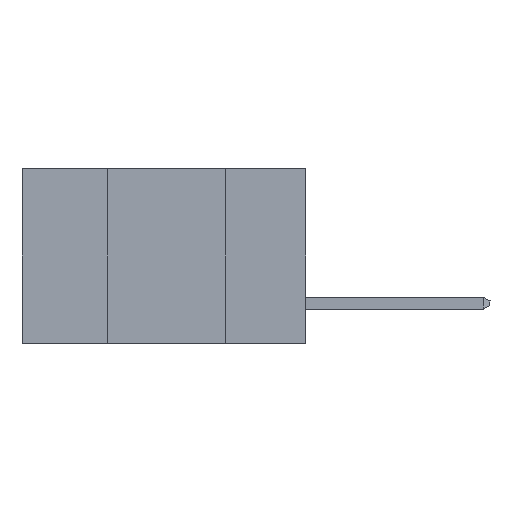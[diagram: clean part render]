
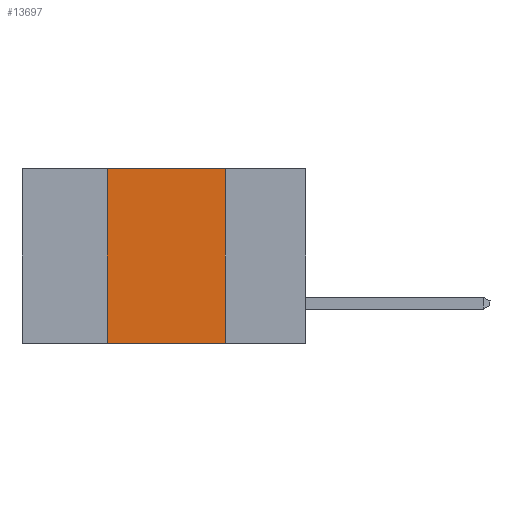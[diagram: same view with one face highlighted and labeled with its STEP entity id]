
A CAD part, left-side view. The second image highlights one B-rep face of the part: STEP entity #13697.
In plain terms, the highlighted planar face has unit normal (-1, 0, 0).
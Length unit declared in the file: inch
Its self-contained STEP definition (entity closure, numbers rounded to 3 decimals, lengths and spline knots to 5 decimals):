
#27 = VECTOR ( 'NONE', #10777, 39.37008 ) ;
#52 = DIRECTION ( 'NONE',  ( 0., -1., 0. ) ) ;
#496 = DIRECTION ( 'NONE',  ( 1., 0., 0. ) ) ;
#500 = DIRECTION ( 'NONE',  ( 0., 0., 1. ) ) ;
#2485 = EDGE_CURVE ( 'NONE', #3078, #5836, #11217, .T. ) ;
#2499 = ORIENTED_EDGE ( 'NONE', *, *, #14195, .F. ) ;
#2854 = VECTOR ( 'NONE', #4933, 39.37008 ) ;
#3003 = AXIS2_PLACEMENT_3D ( 'NONE', #12681, #496, #5812 ) ;
#3078 = VERTEX_POINT ( 'NONE', #17402 ) ;
#3918 = FACE_OUTER_BOUND ( 'NONE', #5797, .T. ) ;
#4214 = CARTESIAN_POINT ( 'NONE',  ( 0., 0.17, -0.37 ) ) ;
#4348 = LINE ( 'NONE', #12487, #27 ) ;
#4933 = DIRECTION ( 'NONE',  ( 0., 0., -1. ) ) ;
#5797 = EDGE_LOOP ( 'NONE', ( #2499, #14328, #10092, #8984 ) ) ;
#5812 = DIRECTION ( 'NONE',  ( 0., 0., -1. ) ) ;
#5836 = VERTEX_POINT ( 'NONE', #7734 ) ;
#6937 = CARTESIAN_POINT ( 'NONE',  ( 0., 0.17, 0. ) ) ;
#7551 = VECTOR ( 'NONE', #500, 39.37008 ) ;
#7584 = CARTESIAN_POINT ( 'NONE',  ( 0., 0.17, 0. ) ) ;
#7734 = CARTESIAN_POINT ( 'NONE',  ( 0., 0.42, 0. ) ) ;
#8492 = VERTEX_POINT ( 'NONE', #6937 ) ;
#8624 = EDGE_CURVE ( 'NONE', #3078, #15073, #16427, .T. ) ;
#8984 = ORIENTED_EDGE ( 'NONE', *, *, #8624, .T. ) ;
#10092 = ORIENTED_EDGE ( 'NONE', *, *, #2485, .F. ) ;
#10193 = LINE ( 'NONE', #7584, #2854 ) ;
#10777 = DIRECTION ( 'NONE',  ( 0., -1., 0. ) ) ;
#11217 = LINE ( 'NONE', #15448, #7551 ) ;
#12487 = CARTESIAN_POINT ( 'NONE',  ( 0., 0.6, 0. ) ) ;
#12681 = CARTESIAN_POINT ( 'NONE',  ( 0., 0.6, 0. ) ) ;
#12752 = VECTOR ( 'NONE', #52, 39.37008 ) ;
#13520 = EDGE_CURVE ( 'NONE', #5836, #8492, #4348, .T. ) ;
#13697 = ADVANCED_FACE ( 'NONE', ( #3918 ), #15686, .F. ) ;
#13834 = CARTESIAN_POINT ( 'NONE',  ( 0., 0.6, -0.37 ) ) ;
#14195 = EDGE_CURVE ( 'NONE', #8492, #15073, #10193, .T. ) ;
#14328 = ORIENTED_EDGE ( 'NONE', *, *, #13520, .F. ) ;
#15073 = VERTEX_POINT ( 'NONE', #4214 ) ;
#15448 = CARTESIAN_POINT ( 'NONE',  ( 0., 0.42, 0. ) ) ;
#15686 = PLANE ( 'NONE',  #3003 ) ;
#16427 = LINE ( 'NONE', #13834, #12752 ) ;
#17402 = CARTESIAN_POINT ( 'NONE',  ( 0., 0.42, -0.37 ) ) ;
